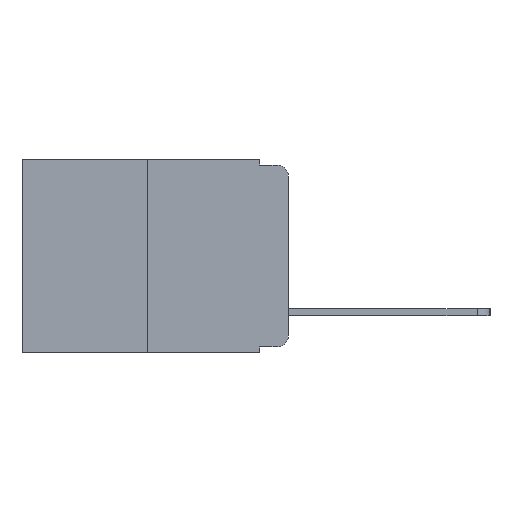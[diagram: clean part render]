
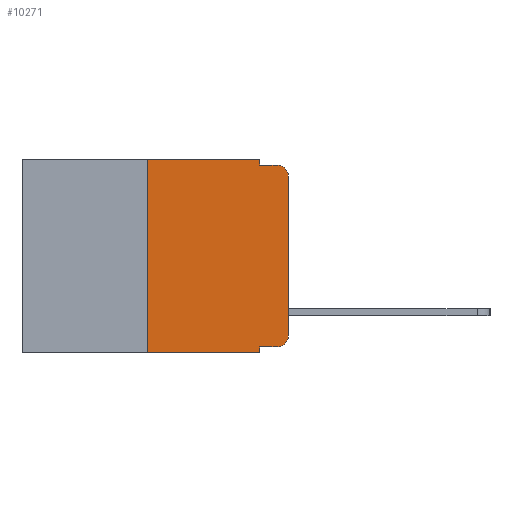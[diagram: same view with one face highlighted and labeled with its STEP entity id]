
A CAD part, left-side view. The second image highlights one B-rep face of the part: STEP entity #10271.
In plain terms, the highlighted planar face has unit normal (-1, 0, 0).
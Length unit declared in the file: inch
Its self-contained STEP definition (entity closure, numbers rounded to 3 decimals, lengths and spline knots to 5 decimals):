
#98 = CARTESIAN_POINT ( 'NONE',  ( 0., 0.02, -0.03 ) ) ;
#282 = VERTEX_POINT ( 'NONE', #3193 ) ;
#686 = ORIENTED_EDGE ( 'NONE', *, *, #7159, .F. ) ;
#1154 = ORIENTED_EDGE ( 'NONE', *, *, #5263, .F. ) ;
#1170 = CARTESIAN_POINT ( 'NONE',  ( 0., 0.02, -0.333 ) ) ;
#1225 = VERTEX_POINT ( 'NONE', #3834 ) ;
#1292 = CARTESIAN_POINT ( 'NONE',  ( 0., 0.051, 0. ) ) ;
#1643 = DIRECTION ( 'NONE',  ( 0., 0., -1. ) ) ;
#1685 = VECTOR ( 'NONE', #16690, 39.37008 ) ;
#1707 = CIRCLE ( 'NONE', #9067, 0.02 ) ;
#1870 = VECTOR ( 'NONE', #8462, 39.37008 ) ;
#1909 = VERTEX_POINT ( 'NONE', #9910 ) ;
#2373 = CARTESIAN_POINT ( 'NONE',  ( 0., 0.25, 0. ) ) ;
#2507 = LINE ( 'NONE', #15926, #2921 ) ;
#2626 = EDGE_CURVE ( 'NONE', #10550, #1225, #4621, .T. ) ;
#2921 = VECTOR ( 'NONE', #4162, 39.37008 ) ;
#2968 = DIRECTION ( 'NONE',  ( 0., -1., 0. ) ) ;
#3066 = DIRECTION ( 'NONE',  ( 0., -1., 0. ) ) ;
#3193 = CARTESIAN_POINT ( 'NONE',  ( 0., 0.25, -0.343 ) ) ;
#3208 = CARTESIAN_POINT ( 'NONE',  ( 0., 0.051, -0.343 ) ) ;
#3511 = EDGE_CURVE ( 'NONE', #11517, #10550, #8914, .T. ) ;
#3554 = CARTESIAN_POINT ( 'NONE',  ( 0., 0.473, 0. ) ) ;
#3834 = CARTESIAN_POINT ( 'NONE',  ( 0., 0., -0.313 ) ) ;
#3900 = CARTESIAN_POINT ( 'NONE',  ( 0., 0.051, 0. ) ) ;
#3907 = ORIENTED_EDGE ( 'NONE', *, *, #8080, .F. ) ;
#3984 = CARTESIAN_POINT ( 'NONE',  ( 0., 0.051, -0.333 ) ) ;
#4162 = DIRECTION ( 'NONE',  ( 0., 0., 1. ) ) ;
#4201 = VERTEX_POINT ( 'NONE', #6875 ) ;
#4254 = DIRECTION ( 'NONE',  ( 0., 0., -1. ) ) ;
#4362 = EDGE_CURVE ( 'NONE', #11517, #5338, #5434, .T. ) ;
#4621 = CIRCLE ( 'NONE', #14143, 0.02 ) ;
#4920 = VECTOR ( 'NONE', #3066, 39.37008 ) ;
#5152 = ORIENTED_EDGE ( 'NONE', *, *, #3511, .T. ) ;
#5263 = EDGE_CURVE ( 'NONE', #282, #6444, #10320, .T. ) ;
#5325 = VECTOR ( 'NONE', #14825, 39.37008 ) ;
#5338 = VERTEX_POINT ( 'NONE', #3208 ) ;
#5434 = LINE ( 'NONE', #3900, #1870 ) ;
#5647 = CARTESIAN_POINT ( 'NONE',  ( 0., 0.473, 0. ) ) ;
#5733 = CARTESIAN_POINT ( 'NONE',  ( 0., 0.051, 0. ) ) ;
#6063 = VERTEX_POINT ( 'NONE', #1292 ) ;
#6286 = DIRECTION ( 'NONE',  ( 0., 0., -1. ) ) ;
#6444 = VERTEX_POINT ( 'NONE', #2373 ) ;
#6875 = CARTESIAN_POINT ( 'NONE',  ( 0., 0.02, -0.01 ) ) ;
#7137 = ORIENTED_EDGE ( 'NONE', *, *, #10765, .T. ) ;
#7159 = EDGE_CURVE ( 'NONE', #6063, #16102, #15344, .T. ) ;
#7316 = CARTESIAN_POINT ( 'NONE',  ( 0., 0.051, -0.01 ) ) ;
#7998 = ORIENTED_EDGE ( 'NONE', *, *, #11706, .F. ) ;
#8080 = EDGE_CURVE ( 'NONE', #16102, #4201, #9838, .T. ) ;
#8427 = ORIENTED_EDGE ( 'NONE', *, *, #15132, .T. ) ;
#8462 = DIRECTION ( 'NONE',  ( 0., 0., -1. ) ) ;
#8609 = LINE ( 'NONE', #11109, #4920 ) ;
#8914 = LINE ( 'NONE', #12932, #1685 ) ;
#8970 = EDGE_CURVE ( 'NONE', #1909, #4201, #1707, .T. ) ;
#9067 = AXIS2_PLACEMENT_3D ( 'NONE', #98, #9787, #1643 ) ;
#9222 = DIRECTION ( 'NONE',  ( 0., 0., 1. ) ) ;
#9399 = VECTOR ( 'NONE', #12056, 39.37008 ) ;
#9580 = AXIS2_PLACEMENT_3D ( 'NONE', #3554, #14044, #6286 ) ;
#9787 = DIRECTION ( 'NONE',  ( -1., 0., 0. ) ) ;
#9838 = LINE ( 'NONE', #15738, #9399 ) ;
#9900 = VECTOR ( 'NONE', #9222, 39.37008 ) ;
#9910 = CARTESIAN_POINT ( 'NONE',  ( 0., 0., -0.03 ) ) ;
#10022 = DIRECTION ( 'NONE',  ( -1., 0., 0. ) ) ;
#10271 = ADVANCED_FACE ( 'NONE', ( #16372 ), #12828, .F. ) ;
#10320 = LINE ( 'NONE', #15306, #9900 ) ;
#10550 = VERTEX_POINT ( 'NONE', #1170 ) ;
#10765 = EDGE_CURVE ( 'NONE', #1225, #1909, #2507, .T. ) ;
#11109 = CARTESIAN_POINT ( 'NONE',  ( 0., 0.473, -0.343 ) ) ;
#11399 = EDGE_LOOP ( 'NONE', ( #7137, #13991, #3907, #686, #7998, #1154, #8427, #15184, #5152, #15569 ) ) ;
#11517 = VERTEX_POINT ( 'NONE', #3984 ) ;
#11706 = EDGE_CURVE ( 'NONE', #6444, #6063, #16144, .T. ) ;
#12056 = DIRECTION ( 'NONE',  ( 0., -1., 0. ) ) ;
#12828 = PLANE ( 'NONE',  #9580 ) ;
#12839 = VECTOR ( 'NONE', #2968, 39.37008 ) ;
#12932 = CARTESIAN_POINT ( 'NONE',  ( 0., 0.051, -0.333 ) ) ;
#13991 = ORIENTED_EDGE ( 'NONE', *, *, #8970, .T. ) ;
#14044 = DIRECTION ( 'NONE',  ( 1., 0., 0. ) ) ;
#14143 = AXIS2_PLACEMENT_3D ( 'NONE', #15628, #10022, #4254 ) ;
#14825 = DIRECTION ( 'NONE',  ( 0., 0., -1. ) ) ;
#15132 = EDGE_CURVE ( 'NONE', #282, #5338, #8609, .T. ) ;
#15184 = ORIENTED_EDGE ( 'NONE', *, *, #4362, .F. ) ;
#15306 = CARTESIAN_POINT ( 'NONE',  ( 0., 0.25, 0. ) ) ;
#15344 = LINE ( 'NONE', #5733, #5325 ) ;
#15569 = ORIENTED_EDGE ( 'NONE', *, *, #2626, .T. ) ;
#15628 = CARTESIAN_POINT ( 'NONE',  ( 0., 0.02, -0.313 ) ) ;
#15738 = CARTESIAN_POINT ( 'NONE',  ( 0., 0.051, -0.01 ) ) ;
#15926 = CARTESIAN_POINT ( 'NONE',  ( 0., 0., 0. ) ) ;
#16102 = VERTEX_POINT ( 'NONE', #7316 ) ;
#16144 = LINE ( 'NONE', #5647, #12839 ) ;
#16372 = FACE_OUTER_BOUND ( 'NONE', #11399, .T. ) ;
#16690 = DIRECTION ( 'NONE',  ( 0., -1., 0. ) ) ;
